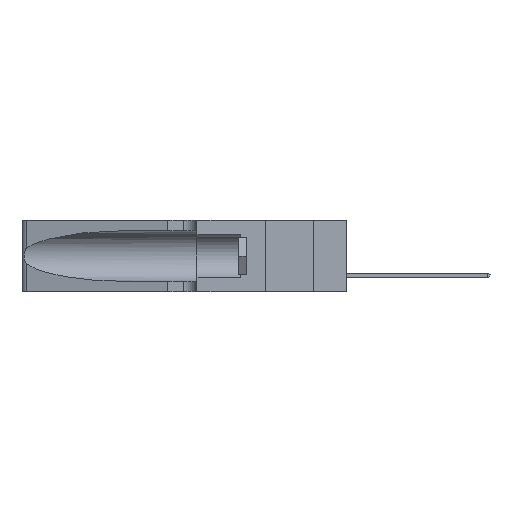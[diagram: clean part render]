
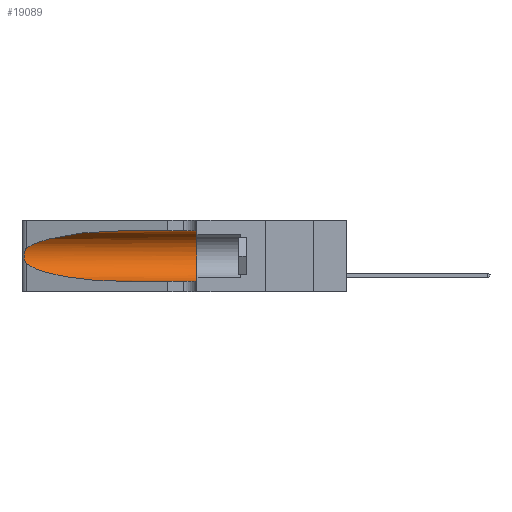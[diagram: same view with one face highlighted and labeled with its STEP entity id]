
A CAD part, left-side view. The second image highlights one B-rep face of the part: STEP entity #19089.
In plain terms, the highlighted cylindrical face has radius 3.308 mm (diameter 6.617 mm), a partial arc.
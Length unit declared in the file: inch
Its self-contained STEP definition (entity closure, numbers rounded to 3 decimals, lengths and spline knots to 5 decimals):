
#1050 = CARTESIAN_POINT ( 'NONE',  ( 0.26018, 1.23835, 0.19895 ) ) ;
#1132 = CARTESIAN_POINT ( 'NONE',  ( 0.25639, 1.23186, 0.15144 ) ) ;
#1152 = FACE_OUTER_BOUND ( 'NONE', #13379, .T. ) ;
#1319 = CARTESIAN_POINT ( 'NONE',  ( 0.18966, 0.96281, 0.31525 ) ) ;
#1567 = CARTESIAN_POINT ( 'NONE',  ( 0.1305, 0.72297, 0.05475 ) ) ;
#1708 = ORIENTED_EDGE ( 'NONE', *, *, #7475, .F. ) ;
#2136 = DIRECTION ( 'NONE',  ( 0., -1., 0. ) ) ;
#2396 = ORIENTED_EDGE ( 'NONE', *, *, #15639, .F. ) ;
#2401 = CARTESIAN_POINT ( 'NONE',  ( 0.25487, 1.22718, 0.14631 ) ) ;
#2589 = VECTOR ( 'NONE', #10002, 39.37008 ) ;
#2799 = CARTESIAN_POINT ( 'NONE',  ( 0.25555, 1.22993, 0.14849 ) ) ;
#2922 = CARTESIAN_POINT ( 'NONE',  ( 0.1305, 0.72297, 0.05475 ) ) ;
#2975 = CARTESIAN_POINT ( 'NONE',  ( 0.26075, 1.23896, 0.178 ) ) ;
#3094 = CARTESIAN_POINT ( 'NONE',  ( 0.1305, 0.72297, 0.31525 ) ) ;
#4011 = VERTEX_POINT ( 'NONE', #24562 ) ;
#4707 = VERTEX_POINT ( 'NONE', #1567 ) ;
#4860 = CARTESIAN_POINT ( 'NONE',  ( 0.25787, 1.23484, 0.2124 ) ) ;
#5333 =( BOUNDED_CURVE ( )  B_SPLINE_CURVE ( 3, ( #19332, #1319, #17287, #15345 ),
 .UNSPECIFIED., .F., .F. ) 
 B_SPLINE_CURVE_WITH_KNOTS ( ( 4, 4 ),
 ( 1.5708, 2.84003 ),
 .UNSPECIFIED. ) 
 CURVE ( )  GEOMETRIC_REPRESENTATION_ITEM ( )  RATIONAL_B_SPLINE_CURVE ( ( 1., 0.87, 0.87, 1. ) ) 
 REPRESENTATION_ITEM ( '' )  );
#5408 = DIRECTION ( 'NONE',  ( 0., 0., 1. ) ) ;
#5999 = CARTESIAN_POINT ( 'NONE',  ( 0.1305, 1.61858, 0.05475 ) ) ;
#7475 = EDGE_CURVE ( 'NONE', #13492, #19713, #18047, .T. ) ;
#7998 = CYLINDRICAL_SURFACE ( 'NONE', #17613, 0.13025 ) ;
#10002 = DIRECTION ( 'NONE',  ( 0., -1., 0. ) ) ;
#10889 = CARTESIAN_POINT ( 'NONE',  ( 0.25789, 1.23486, 0.15765 ) ) ;
#11058 = CARTESIAN_POINT ( 'NONE',  ( 0.25555, 1.22994, 0.2215 ) ) ;
#11087 = B_SPLINE_CURVE_WITH_KNOTS ( 'NONE', 3,
 ( #16844, #11058, #20881, #4860, #22894, #1050, #20796, #2975, #18946, #12959, #10889, #1132, #2799, #16760 ),
 .UNSPECIFIED., .F., .F.,
 ( 4, 2, 2, 2, 2, 2, 4 ),
 ( 0., 0.00027, 0.00053, 0.00107, 0.0016, 0.00187, 0.00214 ),
 .UNSPECIFIED. ) ;
#11253 = CIRCLE ( 'NONE', #24749, 0.13025 ) ;
#11500 = EDGE_CURVE ( 'NONE', #14208, #4707, #25530, .T. ) ;
#11862 = CARTESIAN_POINT ( 'NONE',  ( 0.1305, 1.61858, 0.31525 ) ) ;
#12650 = CARTESIAN_POINT ( 'NONE',  ( 0.25487, 1.22718, 0.14631 ) ) ;
#12959 = CARTESIAN_POINT ( 'NONE',  ( 0.25856, 1.23593, 0.16098 ) ) ;
#13379 = EDGE_LOOP ( 'NONE', ( #19823, #15318, #20101, #18536, #2396, #1708 ) ) ;
#13492 = VERTEX_POINT ( 'NONE', #3094 ) ;
#14208 = VERTEX_POINT ( 'NONE', #2401 ) ;
#14594 = VERTEX_POINT ( 'NONE', #19211 ) ;
#15318 = ORIENTED_EDGE ( 'NONE', *, *, #25363, .T. ) ;
#15345 = CARTESIAN_POINT ( 'NONE',  ( 0.25487, 1.22718, 0.22369 ) ) ;
#15639 = EDGE_CURVE ( 'NONE', #19713, #14594, #11253, .T. ) ;
#16760 = CARTESIAN_POINT ( 'NONE',  ( 0.25487, 1.22718, 0.14631 ) ) ;
#16844 = CARTESIAN_POINT ( 'NONE',  ( 0.25487, 1.22718, 0.22369 ) ) ;
#17287 = CARTESIAN_POINT ( 'NONE',  ( 0.2373, 1.15595, 0.28018 ) ) ;
#17308 = DIRECTION ( 'NONE',  ( 0., 1., 0. ) ) ;
#17402 = CARTESIAN_POINT ( 'NONE',  ( 0.1305, 0.35, 0.185 ) ) ;
#17424 = EDGE_CURVE ( 'NONE', #13492, #4011, #5333, .T. ) ;
#17613 = AXIS2_PLACEMENT_3D ( 'NONE', #20225, #2136, #22401 ) ;
#18047 = LINE ( 'NONE', #11862, #23999 ) ;
#18536 = ORIENTED_EDGE ( 'NONE', *, *, #21200, .T. ) ;
#18538 = LINE ( 'NONE', #5999, #2589 ) ;
#18946 = CARTESIAN_POINT ( 'NONE',  ( 0.26017, 1.23833, 0.17102 ) ) ;
#19089 = ADVANCED_FACE ( 'NONE', ( #1152 ), #7998, .F. ) ;
#19211 = CARTESIAN_POINT ( 'NONE',  ( 0.1305, 0.35, 0.05475 ) ) ;
#19236 = CARTESIAN_POINT ( 'NONE',  ( 0.1305, 0.35, 0.31525 ) ) ;
#19332 = CARTESIAN_POINT ( 'NONE',  ( 0.1305, 0.72297, 0.31525 ) ) ;
#19713 = VERTEX_POINT ( 'NONE', #19236 ) ;
#19823 = ORIENTED_EDGE ( 'NONE', *, *, #17424, .T. ) ;
#20101 = ORIENTED_EDGE ( 'NONE', *, *, #11500, .T. ) ;
#20225 = CARTESIAN_POINT ( 'NONE',  ( 0.1305, 1.61858, 0.185 ) ) ;
#20747 = CARTESIAN_POINT ( 'NONE',  ( 0.2373, 1.15595, 0.08982 ) ) ;
#20796 = CARTESIAN_POINT ( 'NONE',  ( 0.26075, 1.23896, 0.19203 ) ) ;
#20881 = CARTESIAN_POINT ( 'NONE',  ( 0.25639, 1.23184, 0.21858 ) ) ;
#21200 = EDGE_CURVE ( 'NONE', #4707, #14594, #18538, .T. ) ;
#22401 = DIRECTION ( 'NONE',  ( 0., 0., -1. ) ) ;
#22591 = CARTESIAN_POINT ( 'NONE',  ( 0.18966, 0.96281, 0.05475 ) ) ;
#22894 = CARTESIAN_POINT ( 'NONE',  ( 0.25854, 1.2359, 0.20912 ) ) ;
#23999 = VECTOR ( 'NONE', #25878, 39.37008 ) ;
#24562 = CARTESIAN_POINT ( 'NONE',  ( 0.25487, 1.22718, 0.22369 ) ) ;
#24749 = AXIS2_PLACEMENT_3D ( 'NONE', #17402, #17308, #5408 ) ;
#25363 = EDGE_CURVE ( 'NONE', #4011, #14208, #11087, .T. ) ;
#25530 =( BOUNDED_CURVE ( )  B_SPLINE_CURVE ( 3, ( #12650, #20747, #22591, #2922 ),
 .UNSPECIFIED., .F., .T. ) 
 B_SPLINE_CURVE_WITH_KNOTS ( ( 4, 4 ),
 ( 3.44316, 4.71239 ),
 .UNSPECIFIED. ) 
 CURVE ( )  GEOMETRIC_REPRESENTATION_ITEM ( )  RATIONAL_B_SPLINE_CURVE ( ( 1., 0.87, 0.87, 1. ) ) 
 REPRESENTATION_ITEM ( '' )  );
#25878 = DIRECTION ( 'NONE',  ( 0., -1., 0. ) ) ;
